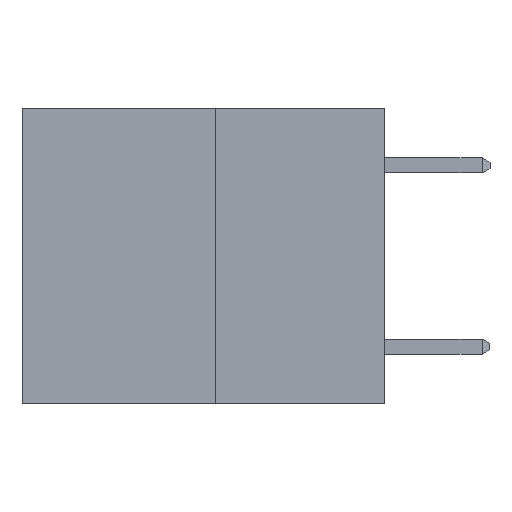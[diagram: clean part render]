
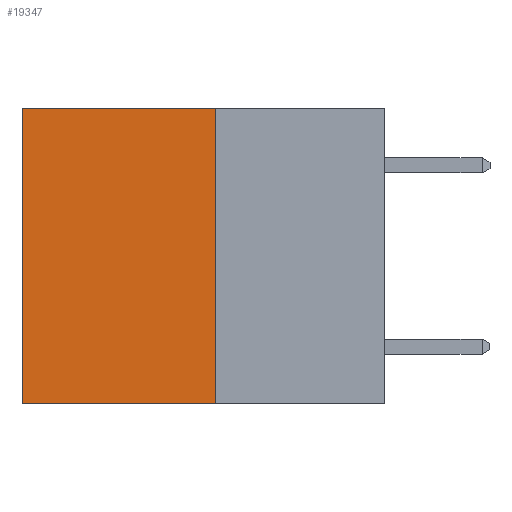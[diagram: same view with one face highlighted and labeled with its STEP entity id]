
A CAD part, left-side view. The second image highlights one B-rep face of the part: STEP entity #19347.
In plain terms, the highlighted planar face has unit normal (-1, 0, 0).
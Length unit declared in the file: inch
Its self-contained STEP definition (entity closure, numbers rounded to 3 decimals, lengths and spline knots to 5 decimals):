
#180 = EDGE_LOOP ( 'NONE', ( #2222, #12587, #2716, #16897 ) ) ;
#296 = AXIS2_PLACEMENT_3D ( 'NONE', #18811, #14138, #15594 ) ;
#2222 = ORIENTED_EDGE ( 'NONE', *, *, #2417, .T. ) ;
#2417 = EDGE_CURVE ( 'NONE', #14001, #17998, #11682, .T. ) ;
#2716 = ORIENTED_EDGE ( 'NONE', *, *, #19182, .F. ) ;
#2915 = VERTEX_POINT ( 'NONE', #19349 ) ;
#3789 = LINE ( 'NONE', #11063, #20067 ) ;
#4062 = VECTOR ( 'NONE', #11896, 39.37008 ) ;
#4564 = CARTESIAN_POINT ( 'NONE',  ( 0.3165, 0.6, -0.49 ) ) ;
#4782 = PLANE ( 'NONE',  #296 ) ;
#6180 = DIRECTION ( 'NONE',  ( 0., 1., 0. ) ) ;
#6231 = EDGE_CURVE ( 'NONE', #2915, #17998, #3789, .T. ) ;
#6471 = CARTESIAN_POINT ( 'NONE',  ( 0.3165, 0.28, -0.49 ) ) ;
#7419 = VERTEX_POINT ( 'NONE', #18669 ) ;
#9675 = LINE ( 'NONE', #14132, #18384 ) ;
#10164 = CARTESIAN_POINT ( 'NONE',  ( 0.3165, 0.6, -0.49 ) ) ;
#11063 = CARTESIAN_POINT ( 'NONE',  ( 0.3165, 0.28, -0.49 ) ) ;
#11213 = DIRECTION ( 'NONE',  ( 0., 1., 0. ) ) ;
#11367 = VECTOR ( 'NONE', #17498, 39.37008 ) ;
#11682 = LINE ( 'NONE', #10164, #4062 ) ;
#11896 = DIRECTION ( 'NONE',  ( 0., 0., -1. ) ) ;
#12125 = LINE ( 'NONE', #6471, #11367 ) ;
#12587 = ORIENTED_EDGE ( 'NONE', *, *, #6231, .F. ) ;
#14001 = VERTEX_POINT ( 'NONE', #16824 ) ;
#14132 = CARTESIAN_POINT ( 'NONE',  ( 0.3165, 0.28, 0. ) ) ;
#14138 = DIRECTION ( 'NONE',  ( 1., 0., 0. ) ) ;
#15594 = DIRECTION ( 'NONE',  ( 0., 0., -1. ) ) ;
#16824 = CARTESIAN_POINT ( 'NONE',  ( 0.3165, 0.6, 0. ) ) ;
#16897 = ORIENTED_EDGE ( 'NONE', *, *, #17268, .T. ) ;
#17268 = EDGE_CURVE ( 'NONE', #7419, #14001, #9675, .T. ) ;
#17498 = DIRECTION ( 'NONE',  ( 0., 0., -1. ) ) ;
#17998 = VERTEX_POINT ( 'NONE', #4564 ) ;
#18384 = VECTOR ( 'NONE', #6180, 39.37008 ) ;
#18669 = CARTESIAN_POINT ( 'NONE',  ( 0.3165, 0.28, 0. ) ) ;
#18811 = CARTESIAN_POINT ( 'NONE',  ( 0.3165, 0.28, -0.49 ) ) ;
#19058 = FACE_OUTER_BOUND ( 'NONE', #180, .T. ) ;
#19182 = EDGE_CURVE ( 'NONE', #7419, #2915, #12125, .T. ) ;
#19347 = ADVANCED_FACE ( 'NONE', ( #19058 ), #4782, .F. ) ;
#19349 = CARTESIAN_POINT ( 'NONE',  ( 0.3165, 0.28, -0.49 ) ) ;
#20067 = VECTOR ( 'NONE', #11213, 39.37008 ) ;
